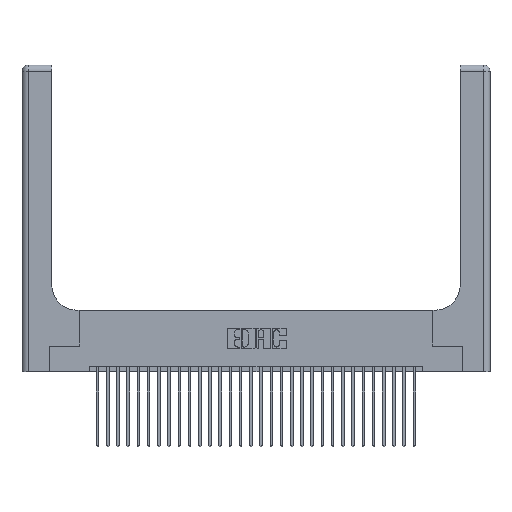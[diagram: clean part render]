
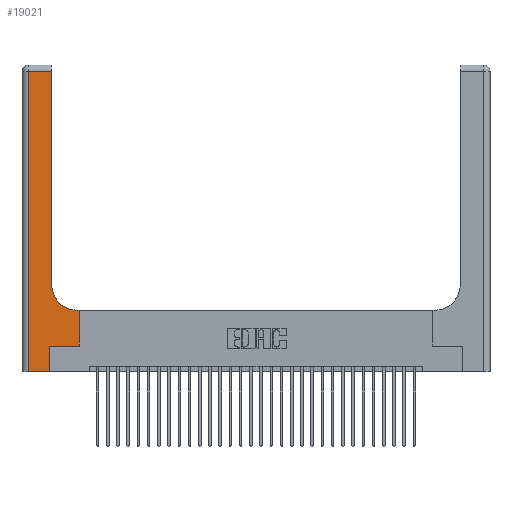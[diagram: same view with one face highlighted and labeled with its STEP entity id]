
A CAD part, top view. The second image highlights one B-rep face of the part: STEP entity #19021.
In plain terms, the highlighted planar face has unit normal (0, 0, 1).
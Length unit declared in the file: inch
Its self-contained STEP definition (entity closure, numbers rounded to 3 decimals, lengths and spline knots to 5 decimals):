
#267 = DIRECTION ( 'NONE',  ( 0., 1., 0. ) ) ;
#799 = VERTEX_POINT ( 'NONE', #20087 ) ;
#1784 = VERTEX_POINT ( 'NONE', #25854 ) ;
#1838 = CARTESIAN_POINT ( 'NONE',  ( 0.5585, 0.6, 0.37 ) ) ;
#2438 = VERTEX_POINT ( 'NONE', #1838 ) ;
#2494 = EDGE_CURVE ( 'NONE', #1784, #13793, #20015, .T. ) ;
#3015 = EDGE_CURVE ( 'NONE', #12285, #799, #17679, .T. ) ;
#3112 = CARTESIAN_POINT ( 'NONE',  ( 0.2915, 3., 0.37 ) ) ;
#3738 = VECTOR ( 'NONE', #9381, 39.37008 ) ;
#4872 = DIRECTION ( 'NONE',  ( -1., 0., 0. ) ) ;
#5381 = VECTOR ( 'NONE', #19264, 39.37008 ) ;
#5690 = VECTOR ( 'NONE', #267, 39.37008 ) ;
#5793 = AXIS2_PLACEMENT_3D ( 'NONE', #24335, #19552, #4872 ) ;
#6317 = LINE ( 'NONE', #23541, #25802 ) ;
#6450 = CARTESIAN_POINT ( 'NONE',  ( 0.5415, 0.85, 0.37 ) ) ;
#6871 = EDGE_LOOP ( 'NONE', ( #9170, #16782, #30300, #7889, #25783, #15562, #17640, #18783, #6902 ) ) ;
#6902 = ORIENTED_EDGE ( 'NONE', *, *, #9557, .T. ) ;
#6908 = CARTESIAN_POINT ( 'NONE',  ( 0.269, 0.25, 0.37 ) ) ;
#7042 = CARTESIAN_POINT ( 'NONE',  ( 0.2915, 0.6, 0.37 ) ) ;
#7261 = LINE ( 'NONE', #16901, #25264 ) ;
#7864 = LINE ( 'NONE', #7042, #14402 ) ;
#7889 = ORIENTED_EDGE ( 'NONE', *, *, #30594, .T. ) ;
#8542 = EDGE_CURVE ( 'NONE', #799, #1784, #18433, .T. ) ;
#8900 = DIRECTION ( 'NONE',  ( 1., 0., 0. ) ) ;
#9170 = ORIENTED_EDGE ( 'NONE', *, *, #3015, .T. ) ;
#9328 = CARTESIAN_POINT ( 'NONE',  ( 0.2915, 0.85, 0.37 ) ) ;
#9381 = DIRECTION ( 'NONE',  ( 1., 0., 0. ) ) ;
#9557 = EDGE_CURVE ( 'NONE', #10563, #12285, #28978, .T. ) ;
#10563 = VERTEX_POINT ( 'NONE', #29545 ) ;
#11141 = VECTOR ( 'NONE', #22687, 39.37008 ) ;
#11902 = FACE_OUTER_BOUND ( 'NONE', #6871, .T. ) ;
#12136 = PLANE ( 'NONE',  #5793 ) ;
#12285 = VERTEX_POINT ( 'NONE', #9328 ) ;
#13793 = VERTEX_POINT ( 'NONE', #31542 ) ;
#14402 = VECTOR ( 'NONE', #21711, 39.37008 ) ;
#14443 = DIRECTION ( 'NONE',  ( 1., 0., 0. ) ) ;
#15059 = EDGE_CURVE ( 'NONE', #2438, #10563, #7864, .T. ) ;
#15562 = ORIENTED_EDGE ( 'NONE', *, *, #28855, .T. ) ;
#16279 = AXIS2_PLACEMENT_3D ( 'NONE', #6450, #23578, #8900 ) ;
#16758 = CARTESIAN_POINT ( 'NONE',  ( 0.06, 3., 0.37 ) ) ;
#16762 = LINE ( 'NONE', #26481, #3738 ) ;
#16779 = CARTESIAN_POINT ( 'NONE',  ( 0., 2.94, 0.37 ) ) ;
#16782 = ORIENTED_EDGE ( 'NONE', *, *, #8542, .T. ) ;
#16901 = CARTESIAN_POINT ( 'NONE',  ( 0.269, 0.25, 0.37 ) ) ;
#17640 = ORIENTED_EDGE ( 'NONE', *, *, #30226, .T. ) ;
#17679 = LINE ( 'NONE', #3112, #11141 ) ;
#18346 = CARTESIAN_POINT ( 'NONE',  ( 0.5585, 0.25, 0.37 ) ) ;
#18433 = LINE ( 'NONE', #16779, #5381 ) ;
#18758 = DIRECTION ( 'NONE',  ( 0., 1., 0. ) ) ;
#18783 = ORIENTED_EDGE ( 'NONE', *, *, #15059, .T. ) ;
#19021 = ADVANCED_FACE ( 'NONE', ( #11902 ), #12136, .F. ) ;
#19250 = VECTOR ( 'NONE', #28886, 39.37008 ) ;
#19264 = DIRECTION ( 'NONE',  ( -1., 0., 0. ) ) ;
#19552 = DIRECTION ( 'NONE',  ( 0., 0., -1. ) ) ;
#20015 = LINE ( 'NONE', #16758, #19250 ) ;
#20021 = VERTEX_POINT ( 'NONE', #18346 ) ;
#20087 = CARTESIAN_POINT ( 'NONE',  ( 0.2915, 2.94, 0.37 ) ) ;
#21249 = CARTESIAN_POINT ( 'NONE',  ( 0.269, 0., 0.37 ) ) ;
#21411 = VERTEX_POINT ( 'NONE', #21249 ) ;
#21711 = DIRECTION ( 'NONE',  ( -1., 0., 0. ) ) ;
#22372 = CARTESIAN_POINT ( 'NONE',  ( 0.5585, 0.25, 0.37 ) ) ;
#22687 = DIRECTION ( 'NONE',  ( 0., 1., 0. ) ) ;
#23541 = CARTESIAN_POINT ( 'NONE',  ( 0.269, 0., 0.37 ) ) ;
#23578 = DIRECTION ( 'NONE',  ( 0., 0., -1. ) ) ;
#24130 = VERTEX_POINT ( 'NONE', #6908 ) ;
#24335 = CARTESIAN_POINT ( 'NONE',  ( 0., 3., 0.37 ) ) ;
#25183 = LINE ( 'NONE', #22372, #5690 ) ;
#25264 = VECTOR ( 'NONE', #14443, 39.37008 ) ;
#25677 = EDGE_CURVE ( 'NONE', #21411, #24130, #6317, .T. ) ;
#25783 = ORIENTED_EDGE ( 'NONE', *, *, #25677, .T. ) ;
#25802 = VECTOR ( 'NONE', #18758, 39.37008 ) ;
#25854 = CARTESIAN_POINT ( 'NONE',  ( 0.06, 2.94, 0.37 ) ) ;
#26481 = CARTESIAN_POINT ( 'NONE',  ( 0., 0., 0.37 ) ) ;
#28855 = EDGE_CURVE ( 'NONE', #24130, #20021, #7261, .T. ) ;
#28886 = DIRECTION ( 'NONE',  ( 0., -1., 0. ) ) ;
#28978 = CIRCLE ( 'NONE', #16279, 0.25 ) ;
#29545 = CARTESIAN_POINT ( 'NONE',  ( 0.5415, 0.6, 0.37 ) ) ;
#30226 = EDGE_CURVE ( 'NONE', #20021, #2438, #25183, .T. ) ;
#30300 = ORIENTED_EDGE ( 'NONE', *, *, #2494, .T. ) ;
#30594 = EDGE_CURVE ( 'NONE', #13793, #21411, #16762, .T. ) ;
#31542 = CARTESIAN_POINT ( 'NONE',  ( 0.06, 0., 0.37 ) ) ;
